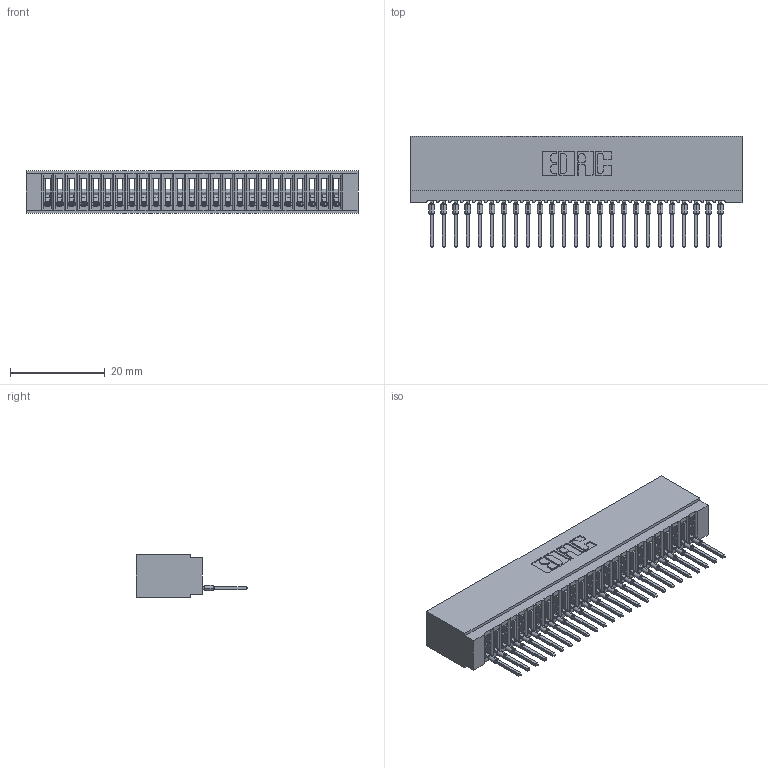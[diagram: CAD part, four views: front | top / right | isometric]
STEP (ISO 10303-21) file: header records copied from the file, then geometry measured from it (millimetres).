
FILE_DESCRIPTION (( 'STEP AP203' ), '1' );
FILE_NAME ('725-025-522-101.STEP', '2026-03-05T21:31:13', ( '' ), ( '' ), 'SwSTEP 2.0', 'SolidWorks 2023', '' );
FILE_SCHEMA (( 'CONFIG_CONTROL_DESIGN' ));
Length unit declared in the file: millimetre
Products named in the file (3): 725 Part_Insulator Option - 01; 725-025-522-101; 745-292-001_522
Assembly tree (26 placements, depth 2):
  725-025-522-101
    725 Part_Insulator Option - 01
    745-292-001_522  x25
Bounding box: 70.1 x 23.51 x 8.89 mm (x, y, z)
Volume: 5426.6 mm3; surface area: 10202 mm2
Topology: 26 solids, 26 shells, 2895 faces, 7954 edges, 5018 vertices
Faces by surface type: plane 1730, cylinder 515, bspline 500, torus 150
Entity records: 43573 total; most frequent: CARTESIAN_POINT 8178, ORIENTED_EDGE 7604, DIRECTION 6610, EDGE_CURVE 3802, LINE 3470, VECTOR 3470, VERTEX_POINT 2426, AXIS2_PLACEMENT_3D 1570
